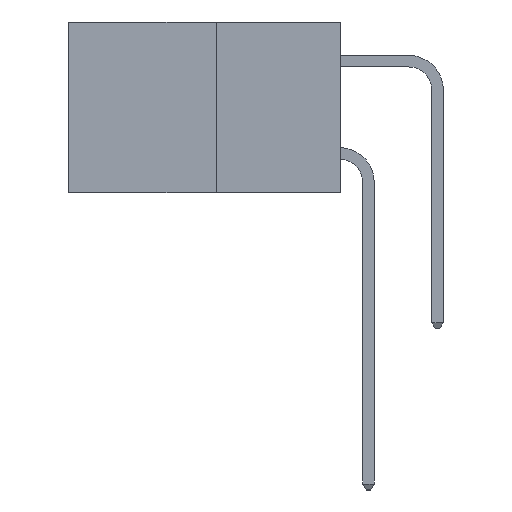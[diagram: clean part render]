
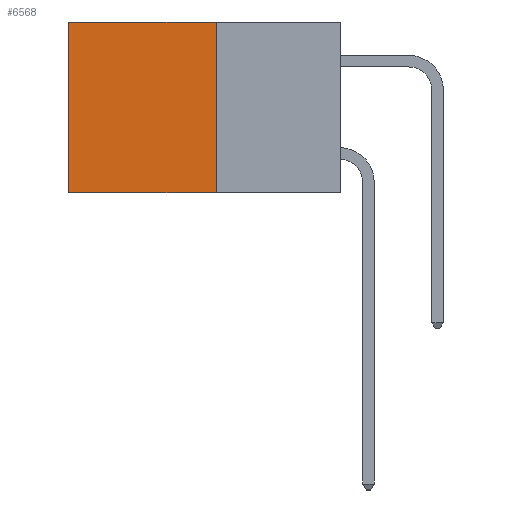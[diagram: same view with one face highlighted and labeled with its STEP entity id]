
A CAD part, left-side view. The second image highlights one B-rep face of the part: STEP entity #6568.
In plain terms, the highlighted planar face has unit normal (-1, 0, 0).
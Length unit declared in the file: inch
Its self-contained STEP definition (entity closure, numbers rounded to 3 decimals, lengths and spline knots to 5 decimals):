
#88 = EDGE_CURVE ( 'NONE', #5783, #6094, #11082, .T. ) ;
#345 = CARTESIAN_POINT ( 'NONE',  ( 0.277, 0.59, -0.37 ) ) ;
#747 = EDGE_CURVE ( 'NONE', #6094, #5032, #11447, .T. ) ;
#1112 = ORIENTED_EDGE ( 'NONE', *, *, #747, .T. ) ;
#1203 = DIRECTION ( 'NONE',  ( 0., 0., -1. ) ) ;
#1850 = FACE_OUTER_BOUND ( 'NONE', #12895, .T. ) ;
#3124 = VERTEX_POINT ( 'NONE', #4788 ) ;
#3178 = DIRECTION ( 'NONE',  ( 0., 0., -1. ) ) ;
#3665 = CARTESIAN_POINT ( 'NONE',  ( 0.277, 0.27, 0. ) ) ;
#4788 = CARTESIAN_POINT ( 'NONE',  ( 0.277, 0.27, -0.37 ) ) ;
#5032 = VERTEX_POINT ( 'NONE', #345 ) ;
#5205 = DIRECTION ( 'NONE',  ( 0., 0., -1. ) ) ;
#5783 = VERTEX_POINT ( 'NONE', #10577 ) ;
#6094 = VERTEX_POINT ( 'NONE', #6579 ) ;
#6568 = ADVANCED_FACE ( 'NONE', ( #1850 ), #10349, .F. ) ;
#6579 = CARTESIAN_POINT ( 'NONE',  ( 0.277, 0.59, 0. ) ) ;
#6867 = ORIENTED_EDGE ( 'NONE', *, *, #11990, .F. ) ;
#7582 = DIRECTION ( 'NONE',  ( 0., 1., 0. ) ) ;
#7990 = ORIENTED_EDGE ( 'NONE', *, *, #88, .T. ) ;
#10349 = PLANE ( 'NONE',  #11119 ) ;
#10577 = CARTESIAN_POINT ( 'NONE',  ( 0.277, 0.27, 0. ) ) ;
#10651 = VECTOR ( 'NONE', #5205, 39.37008 ) ;
#10864 = DIRECTION ( 'NONE',  ( 1., 0., 0. ) ) ;
#10927 = VECTOR ( 'NONE', #7582, 39.37008 ) ;
#11082 = LINE ( 'NONE', #3665, #14561 ) ;
#11119 = AXIS2_PLACEMENT_3D ( 'NONE', #16433, #10864, #1203 ) ;
#11447 = LINE ( 'NONE', #15918, #10651 ) ;
#11990 = EDGE_CURVE ( 'NONE', #3124, #5032, #13999, .T. ) ;
#12110 = LINE ( 'NONE', #16071, #15174 ) ;
#12895 = EDGE_LOOP ( 'NONE', ( #1112, #6867, #16994, #7990 ) ) ;
#12963 = EDGE_CURVE ( 'NONE', #5783, #3124, #12110, .T. ) ;
#13999 = LINE ( 'NONE', #15282, #10927 ) ;
#14561 = VECTOR ( 'NONE', #15825, 39.37008 ) ;
#15174 = VECTOR ( 'NONE', #3178, 39.37008 ) ;
#15282 = CARTESIAN_POINT ( 'NONE',  ( 0.277, 0.27, -0.37 ) ) ;
#15825 = DIRECTION ( 'NONE',  ( 0., 1., 0. ) ) ;
#15918 = CARTESIAN_POINT ( 'NONE',  ( 0.277, 0.59, -0.37 ) ) ;
#16071 = CARTESIAN_POINT ( 'NONE',  ( 0.277, 0.27, -0.37 ) ) ;
#16433 = CARTESIAN_POINT ( 'NONE',  ( 0.277, 0.27, -0.37 ) ) ;
#16994 = ORIENTED_EDGE ( 'NONE', *, *, #12963, .F. ) ;
